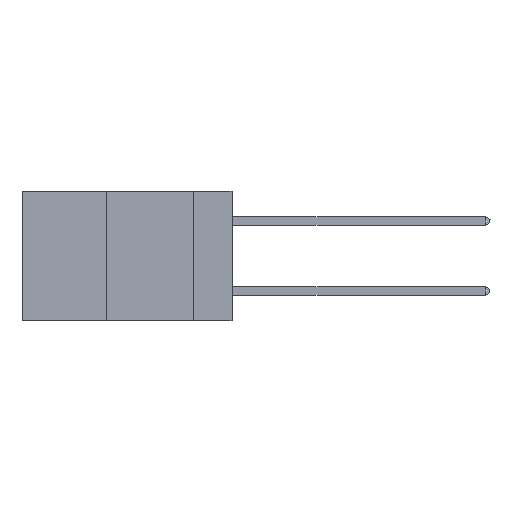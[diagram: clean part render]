
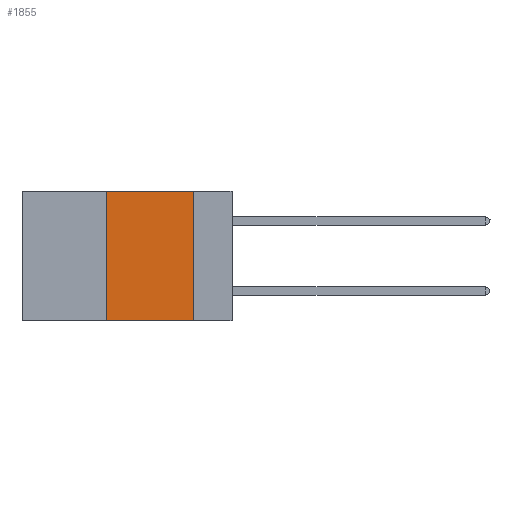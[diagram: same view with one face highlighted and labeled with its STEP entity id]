
A CAD part, left-side view. The second image highlights one B-rep face of the part: STEP entity #1855.
In plain terms, the highlighted planar face has unit normal (-1, 0, 0).
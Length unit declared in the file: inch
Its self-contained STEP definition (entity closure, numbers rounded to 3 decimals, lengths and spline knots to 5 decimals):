
#32 = DIRECTION ( 'NONE',  ( 0., 0., -1. ) ) ;
#1855 = ADVANCED_FACE ( 'NONE', ( #12987 ), #14009, .F. ) ;
#1896 = DIRECTION ( 'NONE',  ( 1., 0., 0. ) ) ;
#4274 = ORIENTED_EDGE ( 'NONE', *, *, #6826, .F. ) ;
#4991 = LINE ( 'NONE', #10796, #17196 ) ;
#5494 = EDGE_CURVE ( 'NONE', #17652, #12898, #4991, .T. ) ;
#5559 = VECTOR ( 'NONE', #21473, 39.37008 ) ;
#6826 = EDGE_CURVE ( 'NONE', #7601, #17652, #10961, .T. ) ;
#7601 = VERTEX_POINT ( 'NONE', #16337 ) ;
#10259 = CARTESIAN_POINT ( 'NONE',  ( 0., 0.36, -0.37 ) ) ;
#10796 = CARTESIAN_POINT ( 'NONE',  ( 0., 0.11, 0. ) ) ;
#10961 = LINE ( 'NONE', #13084, #5559 ) ;
#11681 = VECTOR ( 'NONE', #12259, 39.37008 ) ;
#11891 = AXIS2_PLACEMENT_3D ( 'NONE', #11933, #1896, #14927 ) ;
#11933 = CARTESIAN_POINT ( 'NONE',  ( 0., 0.6, 0. ) ) ;
#12259 = DIRECTION ( 'NONE',  ( 0., 0., 1. ) ) ;
#12540 = CARTESIAN_POINT ( 'NONE',  ( 0., 0.11, 0. ) ) ;
#12774 = VERTEX_POINT ( 'NONE', #10259 ) ;
#12898 = VERTEX_POINT ( 'NONE', #23553 ) ;
#12975 = ORIENTED_EDGE ( 'NONE', *, *, #24350, .F. ) ;
#12987 = FACE_OUTER_BOUND ( 'NONE', #16850, .T. ) ;
#13084 = CARTESIAN_POINT ( 'NONE',  ( 0., 0.6, 0. ) ) ;
#14009 = PLANE ( 'NONE',  #11891 ) ;
#14058 = CARTESIAN_POINT ( 'NONE',  ( 0., 0.36, 0. ) ) ;
#14059 = ORIENTED_EDGE ( 'NONE', *, *, #25583, .T. ) ;
#14927 = DIRECTION ( 'NONE',  ( 0., 0., -1. ) ) ;
#15311 = VECTOR ( 'NONE', #26982, 39.37008 ) ;
#16337 = CARTESIAN_POINT ( 'NONE',  ( 0., 0.36, 0. ) ) ;
#16850 = EDGE_LOOP ( 'NONE', ( #23659, #4274, #12975, #14059 ) ) ;
#17196 = VECTOR ( 'NONE', #32, 39.37008 ) ;
#17652 = VERTEX_POINT ( 'NONE', #12540 ) ;
#20101 = LINE ( 'NONE', #14058, #11681 ) ;
#20471 = CARTESIAN_POINT ( 'NONE',  ( 0., 0.6, -0.37 ) ) ;
#21473 = DIRECTION ( 'NONE',  ( 0., -1., 0. ) ) ;
#23553 = CARTESIAN_POINT ( 'NONE',  ( 0., 0.11, -0.37 ) ) ;
#23659 = ORIENTED_EDGE ( 'NONE', *, *, #5494, .F. ) ;
#24350 = EDGE_CURVE ( 'NONE', #12774, #7601, #20101, .T. ) ;
#25583 = EDGE_CURVE ( 'NONE', #12774, #12898, #27772, .T. ) ;
#26982 = DIRECTION ( 'NONE',  ( 0., -1., 0. ) ) ;
#27772 = LINE ( 'NONE', #20471, #15311 ) ;
